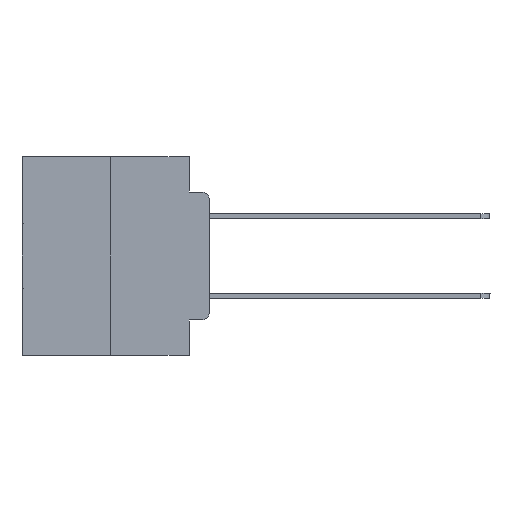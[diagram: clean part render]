
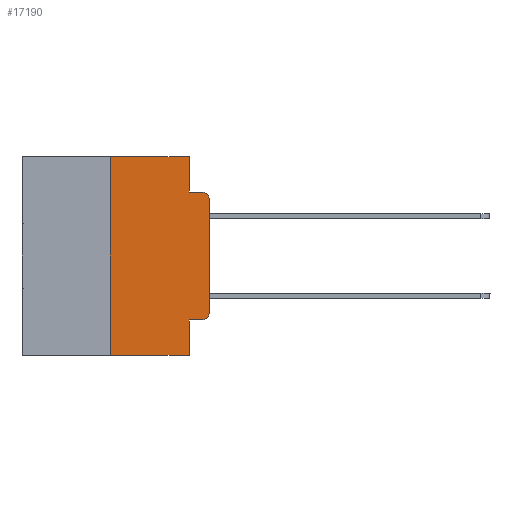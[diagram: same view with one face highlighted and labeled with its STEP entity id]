
A CAD part, left-side view. The second image highlights one B-rep face of the part: STEP entity #17190.
In plain terms, the highlighted planar face has unit normal (-1, 0, 0).
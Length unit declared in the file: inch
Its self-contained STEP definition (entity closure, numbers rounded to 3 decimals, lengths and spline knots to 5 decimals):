
#112 = DIRECTION ( 'NONE',  ( 0., 0., -1. ) ) ;
#513 = CARTESIAN_POINT ( 'NONE',  ( 0., 0.25, 0. ) ) ;
#1079 = CARTESIAN_POINT ( 'NONE',  ( 0., 0.051, 0. ) ) ;
#1250 = CARTESIAN_POINT ( 'NONE',  ( 0., 0.02, -0.4115 ) ) ;
#1557 = CARTESIAN_POINT ( 'NONE',  ( 0., 0.02, -0.0885 ) ) ;
#1602 = CARTESIAN_POINT ( 'NONE',  ( 0., 0.473, -0.5 ) ) ;
#2114 = CARTESIAN_POINT ( 'NONE',  ( 0., 0.051, 0. ) ) ;
#2261 = LINE ( 'NONE', #2114, #25818 ) ;
#2452 = AXIS2_PLACEMENT_3D ( 'NONE', #27290, #24993, #11105 ) ;
#2796 = LINE ( 'NONE', #513, #23719 ) ;
#3042 = VERTEX_POINT ( 'NONE', #18256 ) ;
#3142 = DIRECTION ( 'NONE',  ( 0., 0., 1. ) ) ;
#3531 = CARTESIAN_POINT ( 'NONE',  ( 0., 0.25, -0.5 ) ) ;
#3754 = EDGE_CURVE ( 'NONE', #6800, #9522, #3971, .T. ) ;
#3971 = CIRCLE ( 'NONE', #24888, 0.02 ) ;
#4058 = EDGE_CURVE ( 'NONE', #28034, #14154, #29622, .T. ) ;
#4075 = CARTESIAN_POINT ( 'NONE',  ( 0., 0., -0.3915 ) ) ;
#4156 = LINE ( 'NONE', #18615, #24792 ) ;
#4314 = ORIENTED_EDGE ( 'NONE', *, *, #28193, .T. ) ;
#4737 = LINE ( 'NONE', #25913, #4768 ) ;
#4768 = VECTOR ( 'NONE', #28197, 39.37008 ) ;
#5613 = DIRECTION ( 'NONE',  ( 1., 0., 0. ) ) ;
#5759 = VERTEX_POINT ( 'NONE', #27478 ) ;
#6040 = VERTEX_POINT ( 'NONE', #1079 ) ;
#6395 = EDGE_CURVE ( 'NONE', #9522, #8746, #16389, .T. ) ;
#6618 = CARTESIAN_POINT ( 'NONE',  ( 0., 0.25, 0. ) ) ;
#6800 = VERTEX_POINT ( 'NONE', #1250 ) ;
#7291 = VECTOR ( 'NONE', #19290, 39.37008 ) ;
#7381 = VECTOR ( 'NONE', #10863, 39.37008 ) ;
#7500 = DIRECTION ( 'NONE',  ( 0., 0., 1. ) ) ;
#8020 = ORIENTED_EDGE ( 'NONE', *, *, #4058, .T. ) ;
#8358 = DIRECTION ( 'NONE',  ( 0., 0., -1. ) ) ;
#8725 = ORIENTED_EDGE ( 'NONE', *, *, #16946, .F. ) ;
#8746 = VERTEX_POINT ( 'NONE', #28653 ) ;
#9522 = VERTEX_POINT ( 'NONE', #4075 ) ;
#9538 = EDGE_CURVE ( 'NONE', #3042, #6800, #13796, .T. ) ;
#10003 = LINE ( 'NONE', #24179, #7291 ) ;
#10713 = ORIENTED_EDGE ( 'NONE', *, *, #6395, .T. ) ;
#10863 = DIRECTION ( 'NONE',  ( 0., -1., 0. ) ) ;
#11105 = DIRECTION ( 'NONE',  ( 0., 0., -1. ) ) ;
#11653 = DIRECTION ( 'NONE',  ( -1., 0., 0. ) ) ;
#11816 = EDGE_LOOP ( 'NONE', ( #10713, #4314, #8725, #20014, #29352, #13423, #8020, #16484, #25106, #15068 ) ) ;
#13017 = VERTEX_POINT ( 'NONE', #6618 ) ;
#13423 = ORIENTED_EDGE ( 'NONE', *, *, #16531, .F. ) ;
#13796 = LINE ( 'NONE', #20516, #20785 ) ;
#14154 = VERTEX_POINT ( 'NONE', #16698 ) ;
#14484 = AXIS2_PLACEMENT_3D ( 'NONE', #28926, #5613, #8358 ) ;
#15068 = ORIENTED_EDGE ( 'NONE', *, *, #3754, .T. ) ;
#16389 = LINE ( 'NONE', #25699, #20690 ) ;
#16484 = ORIENTED_EDGE ( 'NONE', *, *, #28559, .F. ) ;
#16531 = EDGE_CURVE ( 'NONE', #28034, #13017, #2796, .T. ) ;
#16698 = CARTESIAN_POINT ( 'NONE',  ( 0., 0.051, -0.5 ) ) ;
#16701 = VERTEX_POINT ( 'NONE', #1557 ) ;
#16946 = EDGE_CURVE ( 'NONE', #5759, #16701, #4737, .T. ) ;
#17190 = ADVANCED_FACE ( 'NONE', ( #29229 ), #28783, .F. ) ;
#18256 = CARTESIAN_POINT ( 'NONE',  ( 0., 0.051, -0.4115 ) ) ;
#18615 = CARTESIAN_POINT ( 'NONE',  ( 0., 0.473, 0. ) ) ;
#18999 = EDGE_CURVE ( 'NONE', #6040, #5759, #10003, .T. ) ;
#19290 = DIRECTION ( 'NONE',  ( 0., 0., -1. ) ) ;
#20014 = ORIENTED_EDGE ( 'NONE', *, *, #18999, .F. ) ;
#20516 = CARTESIAN_POINT ( 'NONE',  ( 0., 0.051, -0.4115 ) ) ;
#20671 = DIRECTION ( 'NONE',  ( 0., 0., -1. ) ) ;
#20690 = VECTOR ( 'NONE', #3142, 39.37008 ) ;
#20785 = VECTOR ( 'NONE', #27403, 39.37008 ) ;
#23354 = DIRECTION ( 'NONE',  ( 0., -1., 0. ) ) ;
#23719 = VECTOR ( 'NONE', #7500, 39.37008 ) ;
#23855 = CIRCLE ( 'NONE', #2452, 0.02 ) ;
#24179 = CARTESIAN_POINT ( 'NONE',  ( 0., 0.051, 0. ) ) ;
#24792 = VECTOR ( 'NONE', #23354, 39.37008 ) ;
#24888 = AXIS2_PLACEMENT_3D ( 'NONE', #27842, #11653, #112 ) ;
#24993 = DIRECTION ( 'NONE',  ( -1., 0., 0. ) ) ;
#25106 = ORIENTED_EDGE ( 'NONE', *, *, #9538, .T. ) ;
#25699 = CARTESIAN_POINT ( 'NONE',  ( 0., 0., 0. ) ) ;
#25818 = VECTOR ( 'NONE', #20671, 39.37008 ) ;
#25913 = CARTESIAN_POINT ( 'NONE',  ( 0., 0.051, -0.0885 ) ) ;
#27290 = CARTESIAN_POINT ( 'NONE',  ( 0., 0.02, -0.1085 ) ) ;
#27403 = DIRECTION ( 'NONE',  ( 0., -1., 0. ) ) ;
#27478 = CARTESIAN_POINT ( 'NONE',  ( 0., 0.051, -0.0885 ) ) ;
#27763 = EDGE_CURVE ( 'NONE', #13017, #6040, #4156, .T. ) ;
#27842 = CARTESIAN_POINT ( 'NONE',  ( 0., 0.02, -0.3915 ) ) ;
#28034 = VERTEX_POINT ( 'NONE', #3531 ) ;
#28193 = EDGE_CURVE ( 'NONE', #8746, #16701, #23855, .T. ) ;
#28197 = DIRECTION ( 'NONE',  ( 0., -1., 0. ) ) ;
#28559 = EDGE_CURVE ( 'NONE', #3042, #14154, #2261, .T. ) ;
#28653 = CARTESIAN_POINT ( 'NONE',  ( 0., 0., -0.1085 ) ) ;
#28783 = PLANE ( 'NONE',  #14484 ) ;
#28926 = CARTESIAN_POINT ( 'NONE',  ( 0., 0.473, 0. ) ) ;
#29229 = FACE_OUTER_BOUND ( 'NONE', #11816, .T. ) ;
#29352 = ORIENTED_EDGE ( 'NONE', *, *, #27763, .F. ) ;
#29622 = LINE ( 'NONE', #1602, #7381 ) ;
